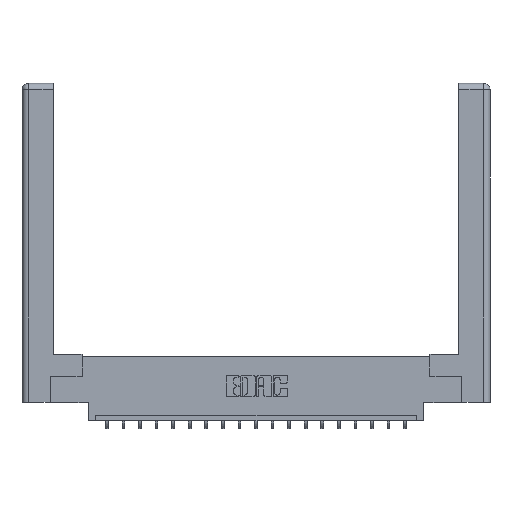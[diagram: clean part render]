
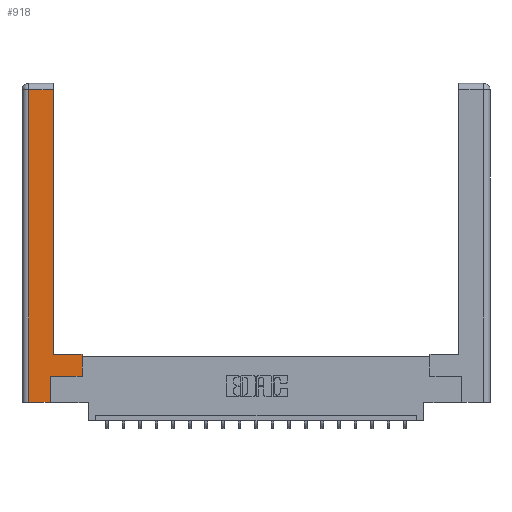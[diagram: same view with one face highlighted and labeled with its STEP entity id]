
A CAD part, top view. The second image highlights one B-rep face of the part: STEP entity #918.
In plain terms, the highlighted planar face has unit normal (0, 0, 1).
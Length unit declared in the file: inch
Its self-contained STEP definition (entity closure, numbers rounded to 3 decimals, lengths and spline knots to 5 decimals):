
#142 = EDGE_CURVE ( 'NONE', #8466, #11960, #8530, .T. ) ;
#430 = CARTESIAN_POINT ( 'NONE',  ( 0., 0., 0. ) ) ;
#918 = ADVANCED_FACE ( 'NONE', ( #18589 ), #18931, .F. ) ;
#946 = ORIENTED_EDGE ( 'NONE', *, *, #16192, .T. ) ;
#1627 = CARTESIAN_POINT ( 'NONE',  ( 0.295, 2.94, 0. ) ) ;
#1696 = CARTESIAN_POINT ( 'NONE',  ( 0.295, 0.45, 0. ) ) ;
#1912 = DIRECTION ( 'NONE',  ( 0., -1., 0. ) ) ;
#2056 = CARTESIAN_POINT ( 'NONE',  ( 0.0615, 0., 0. ) ) ;
#2525 = ORIENTED_EDGE ( 'NONE', *, *, #19042, .T. ) ;
#2572 = CARTESIAN_POINT ( 'NONE',  ( 0.565, 0.45, 0. ) ) ;
#2982 = VECTOR ( 'NONE', #4875, 39.37008 ) ;
#3465 = VECTOR ( 'NONE', #6430, 39.37008 ) ;
#3770 = CARTESIAN_POINT ( 'NONE',  ( 0.295, 0.45, 0. ) ) ;
#3991 = DIRECTION ( 'NONE',  ( -1., 0., 0. ) ) ;
#4174 = LINE ( 'NONE', #1696, #3465 ) ;
#4406 = VECTOR ( 'NONE', #3991, 39.37008 ) ;
#4751 = EDGE_CURVE ( 'NONE', #6118, #14711, #9796, .T. ) ;
#4811 = DIRECTION ( 'NONE',  ( 0., 1., 0. ) ) ;
#4844 = DIRECTION ( 'NONE',  ( -1., 0., 0. ) ) ;
#4875 = DIRECTION ( 'NONE',  ( 1., 0., 0. ) ) ;
#5505 = CARTESIAN_POINT ( 'NONE',  ( 0.565, 0.45, 0. ) ) ;
#5592 = AXIS2_PLACEMENT_3D ( 'NONE', #430, #18870, #4844 ) ;
#5739 = DIRECTION ( 'NONE',  ( 0., 1., 0. ) ) ;
#5753 = ORIENTED_EDGE ( 'NONE', *, *, #11110, .T. ) ;
#6118 = VERTEX_POINT ( 'NONE', #3770 ) ;
#6183 = LINE ( 'NONE', #16384, #18431 ) ;
#6430 = DIRECTION ( 'NONE',  ( -1., 0., 0. ) ) ;
#6567 = CARTESIAN_POINT ( 'NONE',  ( 0.0615, 0., 0. ) ) ;
#6860 = EDGE_CURVE ( 'NONE', #19850, #8466, #11043, .T. ) ;
#7674 = CARTESIAN_POINT ( 'NONE',  ( 0.0615, 2.94, 0. ) ) ;
#7884 = VECTOR ( 'NONE', #14872, 39.37008 ) ;
#7899 = VECTOR ( 'NONE', #5739, 39.37008 ) ;
#7953 = ORIENTED_EDGE ( 'NONE', *, *, #142, .T. ) ;
#8466 = VERTEX_POINT ( 'NONE', #10737 ) ;
#8530 = LINE ( 'NONE', #14047, #2982 ) ;
#8556 = CARTESIAN_POINT ( 'NONE',  ( 0.0615, 2.94, 0. ) ) ;
#9444 = ORIENTED_EDGE ( 'NONE', *, *, #10220, .T. ) ;
#9692 = EDGE_CURVE ( 'NONE', #10048, #6118, #4174, .T. ) ;
#9796 = LINE ( 'NONE', #15003, #17489 ) ;
#10048 = VERTEX_POINT ( 'NONE', #2572 ) ;
#10220 = EDGE_CURVE ( 'NONE', #14711, #10566, #17168, .T. ) ;
#10377 = DIRECTION ( 'NONE',  ( 1., 0., 0. ) ) ;
#10386 = ORIENTED_EDGE ( 'NONE', *, *, #9692, .T. ) ;
#10540 = EDGE_LOOP ( 'NONE', ( #10891, #9444, #5753, #2525, #12507, #7953, #946, #10386 ) ) ;
#10566 = VERTEX_POINT ( 'NONE', #7674 ) ;
#10737 = CARTESIAN_POINT ( 'NONE',  ( 0.265, 0.245, 0. ) ) ;
#10891 = ORIENTED_EDGE ( 'NONE', *, *, #4751, .T. ) ;
#11043 = LINE ( 'NONE', #15097, #7899 ) ;
#11110 = EDGE_CURVE ( 'NONE', #10566, #18817, #16394, .T. ) ;
#11960 = VERTEX_POINT ( 'NONE', #13322 ) ;
#12507 = ORIENTED_EDGE ( 'NONE', *, *, #6860, .T. ) ;
#13322 = CARTESIAN_POINT ( 'NONE',  ( 0.565, 0.245, 0. ) ) ;
#14047 = CARTESIAN_POINT ( 'NONE',  ( 0.565, 0.245, 0. ) ) ;
#14695 = CARTESIAN_POINT ( 'NONE',  ( 0.265, 0., 0. ) ) ;
#14711 = VERTEX_POINT ( 'NONE', #1627 ) ;
#14872 = DIRECTION ( 'NONE',  ( 0., 1., 0. ) ) ;
#15003 = CARTESIAN_POINT ( 'NONE',  ( 0.295, 3., 0. ) ) ;
#15097 = CARTESIAN_POINT ( 'NONE',  ( 0.265, 0.245, 0. ) ) ;
#15208 = VECTOR ( 'NONE', #1912, 39.37008 ) ;
#16192 = EDGE_CURVE ( 'NONE', #11960, #10048, #17051, .T. ) ;
#16384 = CARTESIAN_POINT ( 'NONE',  ( 0.265, 0., 0. ) ) ;
#16394 = LINE ( 'NONE', #6567, #15208 ) ;
#17051 = LINE ( 'NONE', #5505, #7884 ) ;
#17168 = LINE ( 'NONE', #8556, #4406 ) ;
#17489 = VECTOR ( 'NONE', #4811, 39.37008 ) ;
#18431 = VECTOR ( 'NONE', #10377, 39.37008 ) ;
#18589 = FACE_OUTER_BOUND ( 'NONE', #10540, .T. ) ;
#18817 = VERTEX_POINT ( 'NONE', #2056 ) ;
#18870 = DIRECTION ( 'NONE',  ( 0., 0., -1. ) ) ;
#18931 = PLANE ( 'NONE',  #5592 ) ;
#19042 = EDGE_CURVE ( 'NONE', #18817, #19850, #6183, .T. ) ;
#19850 = VERTEX_POINT ( 'NONE', #14695 ) ;
